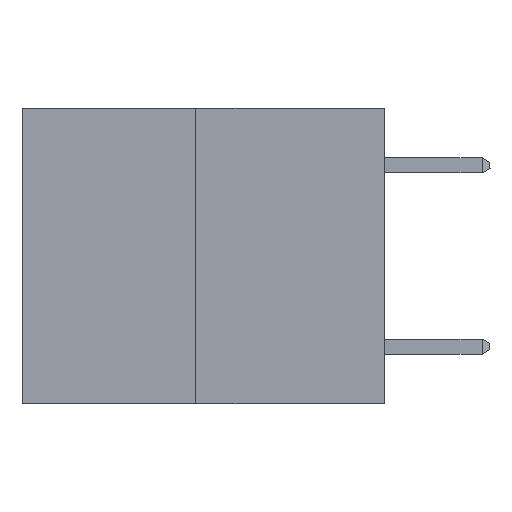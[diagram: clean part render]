
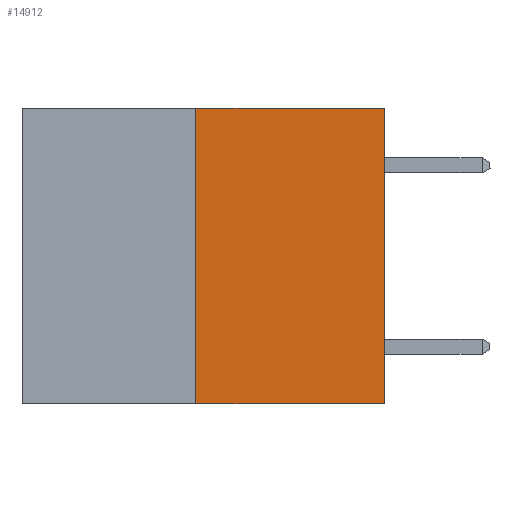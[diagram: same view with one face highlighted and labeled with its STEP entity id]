
A CAD part, left-side view. The second image highlights one B-rep face of the part: STEP entity #14912.
In plain terms, the highlighted planar face has unit normal (-1, 0, 0).
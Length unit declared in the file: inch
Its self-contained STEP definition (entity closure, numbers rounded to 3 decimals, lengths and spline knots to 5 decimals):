
#272 = VECTOR ( 'NONE', #14575, 39.37008 ) ;
#1728 = VECTOR ( 'NONE', #29158, 39.37008 ) ;
#2356 = LINE ( 'NONE', #10663, #6695 ) ;
#6060 = CARTESIAN_POINT ( 'NONE',  ( 0., 0., 0. ) ) ;
#6695 = VECTOR ( 'NONE', #26545, 39.37008 ) ;
#6740 = VERTEX_POINT ( 'NONE', #16595 ) ;
#7909 = CARTESIAN_POINT ( 'NONE',  ( 0., 0.312, -0.49 ) ) ;
#9497 = ORIENTED_EDGE ( 'NONE', *, *, #13242, .F. ) ;
#9820 = DIRECTION ( 'NONE',  ( 0., 0., -1. ) ) ;
#10275 = AXIS2_PLACEMENT_3D ( 'NONE', #16695, #21300, #9820 ) ;
#10663 = CARTESIAN_POINT ( 'NONE',  ( 0., 0.6, -0.49 ) ) ;
#10733 = ORIENTED_EDGE ( 'NONE', *, *, #19215, .T. ) ;
#13206 = EDGE_CURVE ( 'NONE', #29411, #25869, #16872, .T. ) ;
#13207 = CARTESIAN_POINT ( 'NONE',  ( 0., 0.6, 0. ) ) ;
#13242 = EDGE_CURVE ( 'NONE', #6740, #29411, #26534, .T. ) ;
#13341 = LINE ( 'NONE', #6060, #19809 ) ;
#14242 = EDGE_CURVE ( 'NONE', #6740, #18305, #2356, .T. ) ;
#14575 = DIRECTION ( 'NONE',  ( 0., 0., 1. ) ) ;
#14695 = CARTESIAN_POINT ( 'NONE',  ( 0., 0.312, 0. ) ) ;
#14754 = CARTESIAN_POINT ( 'NONE',  ( 0., 0., 0. ) ) ;
#14813 = ORIENTED_EDGE ( 'NONE', *, *, #13206, .F. ) ;
#14912 = ADVANCED_FACE ( 'NONE', ( #26795 ), #28094, .F. ) ;
#15688 = CARTESIAN_POINT ( 'NONE',  ( 0., 0., -0.49 ) ) ;
#16595 = CARTESIAN_POINT ( 'NONE',  ( 0., 0.312, -0.49 ) ) ;
#16695 = CARTESIAN_POINT ( 'NONE',  ( 0., 0.6, 0. ) ) ;
#16872 = LINE ( 'NONE', #13207, #1728 ) ;
#18305 = VERTEX_POINT ( 'NONE', #15688 ) ;
#19215 = EDGE_CURVE ( 'NONE', #18305, #25869, #13341, .T. ) ;
#19809 = VECTOR ( 'NONE', #21202, 39.37008 ) ;
#21009 = EDGE_LOOP ( 'NONE', ( #9497, #28055, #10733, #14813 ) ) ;
#21202 = DIRECTION ( 'NONE',  ( 0., 0., 1. ) ) ;
#21300 = DIRECTION ( 'NONE',  ( 1., 0., 0. ) ) ;
#25869 = VERTEX_POINT ( 'NONE', #14754 ) ;
#26534 = LINE ( 'NONE', #7909, #272 ) ;
#26545 = DIRECTION ( 'NONE',  ( 0., -1., 0. ) ) ;
#26795 = FACE_OUTER_BOUND ( 'NONE', #21009, .T. ) ;
#28055 = ORIENTED_EDGE ( 'NONE', *, *, #14242, .T. ) ;
#28094 = PLANE ( 'NONE',  #10275 ) ;
#29158 = DIRECTION ( 'NONE',  ( 0., -1., 0. ) ) ;
#29411 = VERTEX_POINT ( 'NONE', #14695 ) ;
